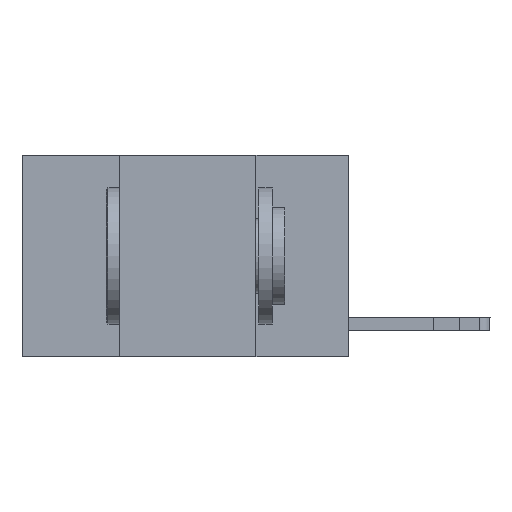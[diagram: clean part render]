
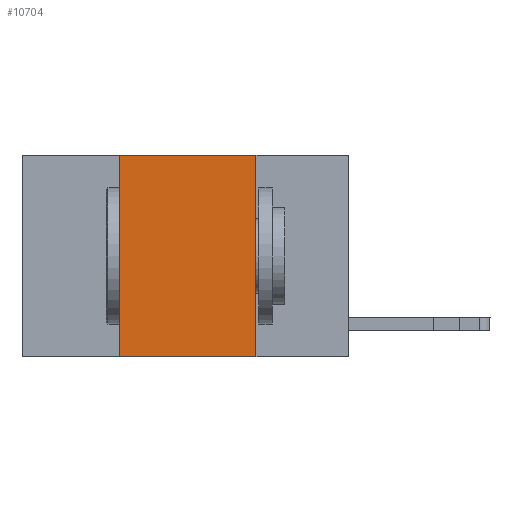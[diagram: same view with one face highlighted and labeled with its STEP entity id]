
A CAD part, left-side view. The second image highlights one B-rep face of the part: STEP entity #10704.
In plain terms, the highlighted planar face has unit normal (-1, 0, 0).
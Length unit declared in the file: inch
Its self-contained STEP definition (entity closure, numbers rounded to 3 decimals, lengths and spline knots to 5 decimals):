
#1479 = LINE ( 'NONE', #2591, #20172 ) ;
#2287 = DIRECTION ( 'NONE',  ( 0., 0., 1. ) ) ;
#2591 = CARTESIAN_POINT ( 'NONE',  ( 0., 0.6, -0.37 ) ) ;
#2905 = ORIENTED_EDGE ( 'NONE', *, *, #12473, .F. ) ;
#3124 = EDGE_CURVE ( 'NONE', #19320, #7679, #4525, .T. ) ;
#3437 = CARTESIAN_POINT ( 'NONE',  ( 0., 0.42, 0. ) ) ;
#3765 = EDGE_CURVE ( 'NONE', #19320, #6539, #1479, .T. ) ;
#4111 = ORIENTED_EDGE ( 'NONE', *, *, #3765, .T. ) ;
#4525 = LINE ( 'NONE', #3437, #23726 ) ;
#5831 = EDGE_LOOP ( 'NONE', ( #16467, #2905, #13725, #4111 ) ) ;
#6539 = VERTEX_POINT ( 'NONE', #19633 ) ;
#7414 = PLANE ( 'NONE',  #15373 ) ;
#7679 = VERTEX_POINT ( 'NONE', #19001 ) ;
#8486 = CARTESIAN_POINT ( 'NONE',  ( 0., 0.17, 0. ) ) ;
#8667 = CARTESIAN_POINT ( 'NONE',  ( 0., 0.6, 0. ) ) ;
#8793 = LINE ( 'NONE', #8667, #19036 ) ;
#9095 = CARTESIAN_POINT ( 'NONE',  ( 0., 0.17, 0. ) ) ;
#10148 = VECTOR ( 'NONE', #23779, 39.37008 ) ;
#10602 = DIRECTION ( 'NONE',  ( 0., -1., 0. ) ) ;
#10704 = ADVANCED_FACE ( 'NONE', ( #24126 ), #7414, .F. ) ;
#11289 = DIRECTION ( 'NONE',  ( 0., 0., -1. ) ) ;
#12473 = EDGE_CURVE ( 'NONE', #7679, #16087, #8793, .T. ) ;
#13725 = ORIENTED_EDGE ( 'NONE', *, *, #3124, .F. ) ;
#13839 = CARTESIAN_POINT ( 'NONE',  ( 0., 0.42, -0.37 ) ) ;
#15243 = LINE ( 'NONE', #8486, #10148 ) ;
#15373 = AXIS2_PLACEMENT_3D ( 'NONE', #20871, #22770, #11289 ) ;
#16087 = VERTEX_POINT ( 'NONE', #9095 ) ;
#16467 = ORIENTED_EDGE ( 'NONE', *, *, #19431, .F. ) ;
#18005 = DIRECTION ( 'NONE',  ( 0., -1., 0. ) ) ;
#19001 = CARTESIAN_POINT ( 'NONE',  ( 0., 0.42, 0. ) ) ;
#19036 = VECTOR ( 'NONE', #10602, 39.37008 ) ;
#19320 = VERTEX_POINT ( 'NONE', #13839 ) ;
#19431 = EDGE_CURVE ( 'NONE', #16087, #6539, #15243, .T. ) ;
#19633 = CARTESIAN_POINT ( 'NONE',  ( 0., 0.17, -0.37 ) ) ;
#20172 = VECTOR ( 'NONE', #18005, 39.37008 ) ;
#20871 = CARTESIAN_POINT ( 'NONE',  ( 0., 0.6, 0. ) ) ;
#22770 = DIRECTION ( 'NONE',  ( 1., 0., 0. ) ) ;
#23726 = VECTOR ( 'NONE', #2287, 39.37008 ) ;
#23779 = DIRECTION ( 'NONE',  ( 0., 0., -1. ) ) ;
#24126 = FACE_OUTER_BOUND ( 'NONE', #5831, .T. ) ;
